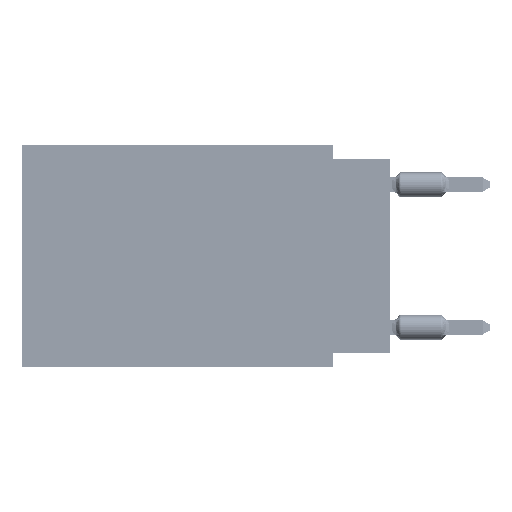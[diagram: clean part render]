
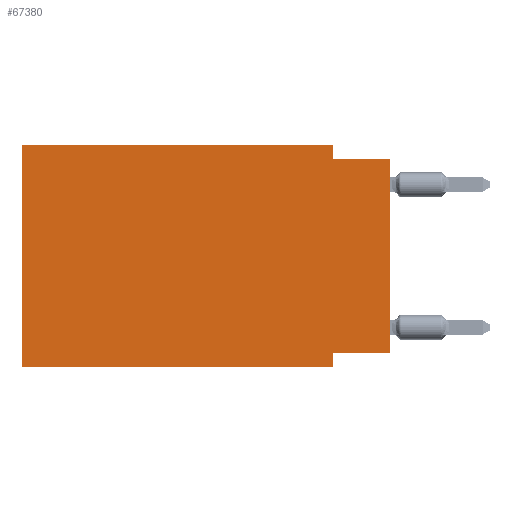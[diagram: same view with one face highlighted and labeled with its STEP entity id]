
A CAD part, left-side view. The second image highlights one B-rep face of the part: STEP entity #67380.
In plain terms, the highlighted planar face has unit normal (-1, 0, 0).
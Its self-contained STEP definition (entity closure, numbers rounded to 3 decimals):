
#905 = ORIENTED_EDGE ( 'NONE', *, *, #68398, .F. ) ;
#2228 = CARTESIAN_POINT ( 'NONE',  ( 0., 0., -9.271 ) ) ;
#4178 = DIRECTION ( 'NONE',  ( 1., 0., 0. ) ) ;
#4540 = EDGE_CURVE ( 'NONE', #38240, #52730, #9703, .T. ) ;
#4810 = ORIENTED_EDGE ( 'NONE', *, *, #13854, .F. ) ;
#4882 = VERTEX_POINT ( 'NONE', #53731 ) ;
#9377 = PLANE ( 'NONE',  #56814 ) ;
#9504 = CARTESIAN_POINT ( 'NONE',  ( 0., 0., 0. ) ) ;
#9566 = EDGE_CURVE ( 'NONE', #55999, #14576, #15424, .T. ) ;
#9703 = LINE ( 'NONE', #14899, #62542 ) ;
#10022 = DIRECTION ( 'NONE',  ( 0., 0., 1. ) ) ;
#11408 = CARTESIAN_POINT ( 'NONE',  ( 0., 16.383, 0. ) ) ;
#12547 = VECTOR ( 'NONE', #36317, 1000. ) ;
#13309 = CARTESIAN_POINT ( 'NONE',  ( 0., 2.54, -9.271 ) ) ;
#13359 = VERTEX_POINT ( 'NONE', #71927 ) ;
#13854 = EDGE_CURVE ( 'NONE', #39705, #4882, #37036, .T. ) ;
#14576 = VERTEX_POINT ( 'NONE', #53531 ) ;
#14899 = CARTESIAN_POINT ( 'NONE',  ( 0., 2.54, -9.906 ) ) ;
#15260 = DIRECTION ( 'NONE',  ( 0., 0., -1. ) ) ;
#15424 = LINE ( 'NONE', #9504, #18173 ) ;
#15470 = DIRECTION ( 'NONE',  ( 0., 0., -1. ) ) ;
#18173 = VECTOR ( 'NONE', #26531, 1000. ) ;
#18619 = LINE ( 'NONE', #41244, #33107 ) ;
#18942 = ORIENTED_EDGE ( 'NONE', *, *, #4540, .F. ) ;
#23527 = CARTESIAN_POINT ( 'NONE',  ( 0., 16.383, -9.906 ) ) ;
#24217 = EDGE_LOOP ( 'NONE', ( #71077, #33335, #42922, #4810, #905, #46948, #18942, #50109 ) ) ;
#24869 = CARTESIAN_POINT ( 'NONE',  ( 0., 2.54, 0. ) ) ;
#25147 = LINE ( 'NONE', #54034, #30554 ) ;
#26418 = DIRECTION ( 'NONE',  ( 0., 0., -1. ) ) ;
#26531 = DIRECTION ( 'NONE',  ( 0., 0., 1. ) ) ;
#29584 = VECTOR ( 'NONE', #10022, 1000. ) ;
#29692 = VERTEX_POINT ( 'NONE', #23527 ) ;
#30554 = VECTOR ( 'NONE', #64446, 1000. ) ;
#33107 = VECTOR ( 'NONE', #63834, 1000. ) ;
#33335 = ORIENTED_EDGE ( 'NONE', *, *, #38395, .F. ) ;
#36317 = DIRECTION ( 'NONE',  ( 0., 1., 0. ) ) ;
#37036 = LINE ( 'NONE', #48521, #58629 ) ;
#38240 = VERTEX_POINT ( 'NONE', #13309 ) ;
#38395 = EDGE_CURVE ( 'NONE', #13359, #14576, #25147, .T. ) ;
#39705 = VERTEX_POINT ( 'NONE', #11408 ) ;
#41244 = CARTESIAN_POINT ( 'NONE',  ( 0., 16.383, -9.906 ) ) ;
#42922 = ORIENTED_EDGE ( 'NONE', *, *, #51932, .F. ) ;
#46948 = ORIENTED_EDGE ( 'NONE', *, *, #63882, .T. ) ;
#48521 = CARTESIAN_POINT ( 'NONE',  ( 0., 16.383, 0. ) ) ;
#50051 = CARTESIAN_POINT ( 'NONE',  ( 0., 16.383, 0. ) ) ;
#50109 = ORIENTED_EDGE ( 'NONE', *, *, #59543, .F. ) ;
#51932 = EDGE_CURVE ( 'NONE', #4882, #13359, #64169, .T. ) ;
#52338 = CARTESIAN_POINT ( 'NONE',  ( 0., 2.54, -9.906 ) ) ;
#52730 = VERTEX_POINT ( 'NONE', #52338 ) ;
#53531 = CARTESIAN_POINT ( 'NONE',  ( 0., 0., -0.635 ) ) ;
#53731 = CARTESIAN_POINT ( 'NONE',  ( 0., 2.54, 0. ) ) ;
#53853 = FACE_OUTER_BOUND ( 'NONE', #24217, .T. ) ;
#54034 = CARTESIAN_POINT ( 'NONE',  ( 0., 0., -0.635 ) ) ;
#54574 = CARTESIAN_POINT ( 'NONE',  ( 0., 16.383, 0. ) ) ;
#55999 = VERTEX_POINT ( 'NONE', #56266 ) ;
#56266 = CARTESIAN_POINT ( 'NONE',  ( 0., 0., -9.271 ) ) ;
#56814 = AXIS2_PLACEMENT_3D ( 'NONE', #54574, #4178, #26418 ) ;
#58629 = VECTOR ( 'NONE', #71475, 1000. ) ;
#59543 = EDGE_CURVE ( 'NONE', #55999, #38240, #64841, .T. ) ;
#60333 = VECTOR ( 'NONE', #15470, 1000. ) ;
#62542 = VECTOR ( 'NONE', #15260, 1000. ) ;
#63834 = DIRECTION ( 'NONE',  ( 0., -1., 0. ) ) ;
#63882 = EDGE_CURVE ( 'NONE', #29692, #52730, #18619, .T. ) ;
#64169 = LINE ( 'NONE', #24869, #60333 ) ;
#64446 = DIRECTION ( 'NONE',  ( 0., -1., 0. ) ) ;
#64841 = LINE ( 'NONE', #2228, #12547 ) ;
#66730 = LINE ( 'NONE', #50051, #29584 ) ;
#67380 = ADVANCED_FACE ( 'NONE', ( #53853 ), #9377, .F. ) ;
#68398 = EDGE_CURVE ( 'NONE', #29692, #39705, #66730, .T. ) ;
#71077 = ORIENTED_EDGE ( 'NONE', *, *, #9566, .T. ) ;
#71475 = DIRECTION ( 'NONE',  ( 0., -1., 0. ) ) ;
#71927 = CARTESIAN_POINT ( 'NONE',  ( 0., 2.54, -0.635 ) ) ;
